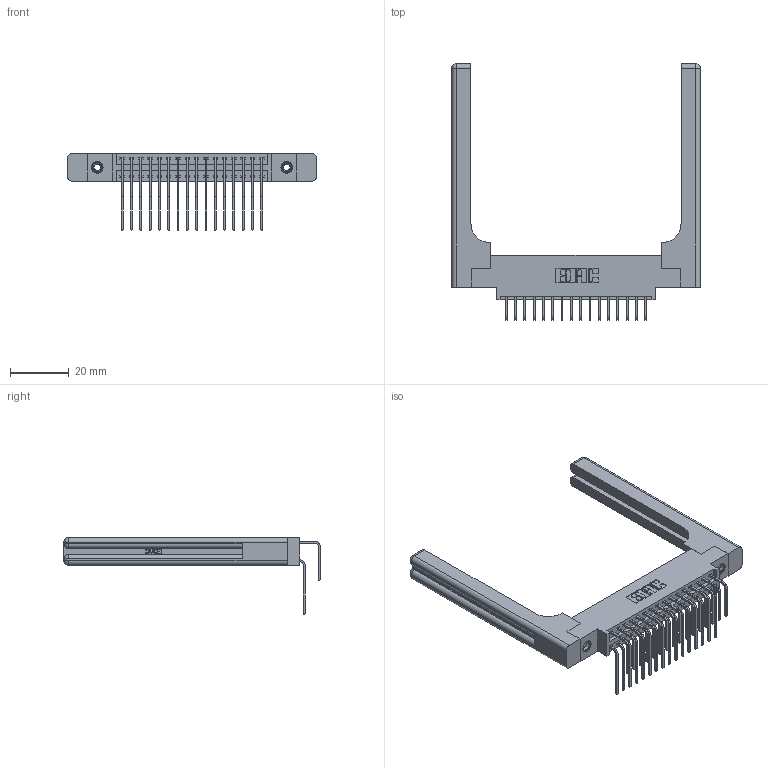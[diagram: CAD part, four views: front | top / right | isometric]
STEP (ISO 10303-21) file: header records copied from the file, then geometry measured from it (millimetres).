
FILE_DESCRIPTION (( 'STEP AP203' ), '1' );
FILE_NAME ('346-032-558-858.STEP', '2022-05-19T18:38:59', ( '' ), ( '' ), 'SwSTEP 2.0', 'SolidWorks 2020', '' );
FILE_SCHEMA (( 'CONFIG_CONTROL_DESIGN' ));
Length unit declared in the file: inch
Products named in the file (6): 346-220-058_345-220-058; 345-250-001_345-250-001-102; 346-032-558-858; 345-292-001_558 Tail - 2; 346 Part_0.170 Offset - 0.156 Dia-TH; 345-292-001_558 559 Tail - 1
Assembly tree (37 placements, depth 2):
  346-032-558-858
    346 Part_0.170 Offset - 0.156 Dia-TH
    345-292-001_558 559 Tail - 1  x16
    345-292-001_558 Tail - 2  x16
    345-250-001_345-250-001-102  x2
    346-220-058_345-220-058  x2
Bounding box: 84.86 x 87.44 x 26.16 mm (x, y, z)
Volume: 15579.2 mm3; surface area: 16777.2 mm2
Topology: 37 solids, 37 shells, 2124 faces, 6195 edges, 4066 vertices
Faces by surface type: plane 1426, cylinder 638, bspline 36, cone 12, sphere 8, torus 4
Entity records: 21456 total; most frequent: CARTESIAN_POINT 4638, ORIENTED_EDGE 3316, DIRECTION 3042, EDGE_CURVE 1658, LINE 1330, VECTOR 1330, VERTEX_POINT 1094, AXIS2_PLACEMENT_3D 856
